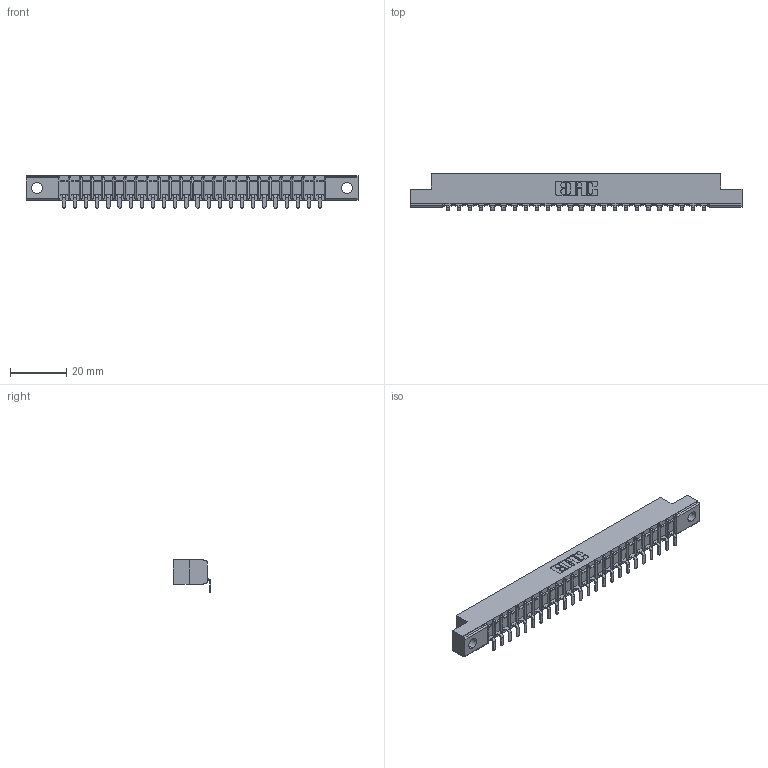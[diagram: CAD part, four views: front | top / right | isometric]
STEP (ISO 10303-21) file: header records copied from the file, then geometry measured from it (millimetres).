
FILE_DESCRIPTION (( 'STEP AP203' ), '1' );
FILE_NAME ('307-024-553-104.STEP', '2018-08-04T06:33:35', ( '' ), ( '' ), 'SwSTEP 2.0', 'SolidWorks 2016', '' );
FILE_SCHEMA (( 'CONFIG_CONTROL_DESIGN' ));
Length unit declared in the file: inch
Products named in the file (3): 307 Part_.156 Dia Mounting Holes; 307-290-002_553; 307-024-553-104
Assembly tree (25 placements, depth 2):
  307-024-553-104
    307 Part_.156 Dia Mounting Holes
    307-290-002_553  x24
Bounding box: 118.11 x 13.32 x 11.51 mm (x, y, z)
Volume: 7692.4 mm3; surface area: 14000.4 mm2
Topology: 25 solids, 25 shells, 2029 faces, 6215 edges, 4074 vertices
Faces by surface type: plane 1212, cylinder 767, sphere 50
Entity records: 24066 total; most frequent: CARTESIAN_POINT 4062, ORIENTED_EDGE 4050, DIRECTION 3947, EDGE_CURVE 2025, VECTOR 1549, LINE 1549, VERTEX_POINT 1314, AXIS2_PLACEMENT_3D 1199
